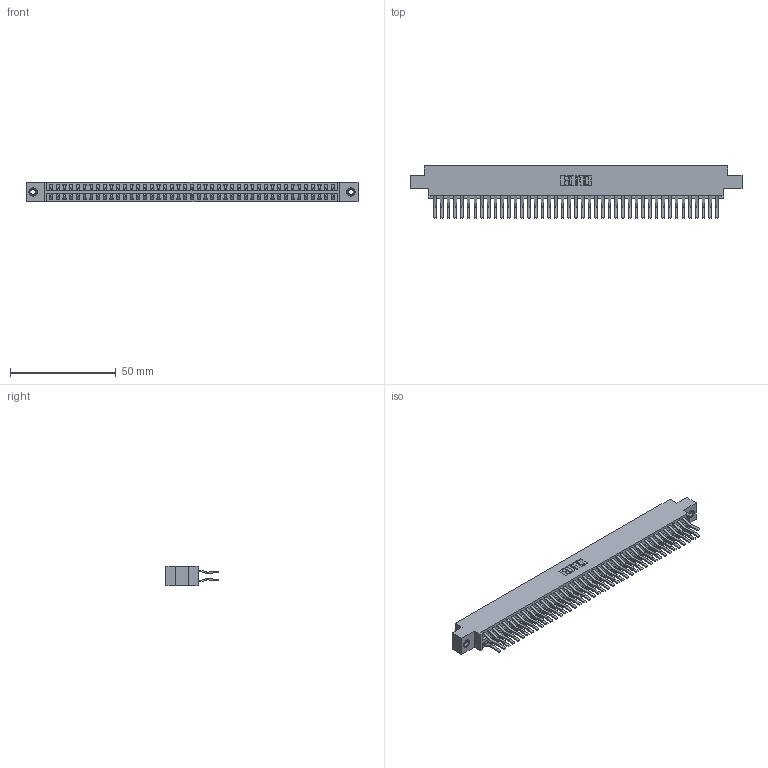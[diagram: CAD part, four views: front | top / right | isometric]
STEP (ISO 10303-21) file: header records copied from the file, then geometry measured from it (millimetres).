
FILE_DESCRIPTION (( 'STEP AP203' ), '1' );
FILE_NAME ('396-086-560-808.STEP', '2019-11-02T14:57:22', ( '' ), ( '' ), 'SwSTEP 2.0', 'SolidWorks 2016', '' );
FILE_SCHEMA (( 'CONFIG_CONTROL_DESIGN' ));
Length unit declared in the file: inch
Products named in the file (4): 396-086-560-808; 346 Part_0.170 Offset - 0.156 Dia-TI; 345-292-001_560 Tail; 345-250-001_345-250-003-102
Assembly tree (89 placements, depth 2):
  396-086-560-808
    346 Part_0.170 Offset - 0.156 Dia-TI
    345-292-001_560 Tail  x86
    345-250-001_345-250-003-102  x2
Bounding box: 157.1 x 24.78 x 9.4 mm (x, y, z)
Volume: 15729.4 mm3; surface area: 23340.5 mm2
Topology: 89 solids, 89 shells, 4830 faces, 14323 edges, 9426 vertices
Faces by surface type: plane 3122, cylinder 1692, cone 12, torus 4
Entity records: 29334 total; most frequent: CARTESIAN_POINT 4819, ORIENTED_EDGE 4746, DIRECTION 4327, EDGE_CURVE 2373, LINE 2045, VECTOR 2045, VERTEX_POINT 1576, AXIS2_PLACEMENT_3D 1141
